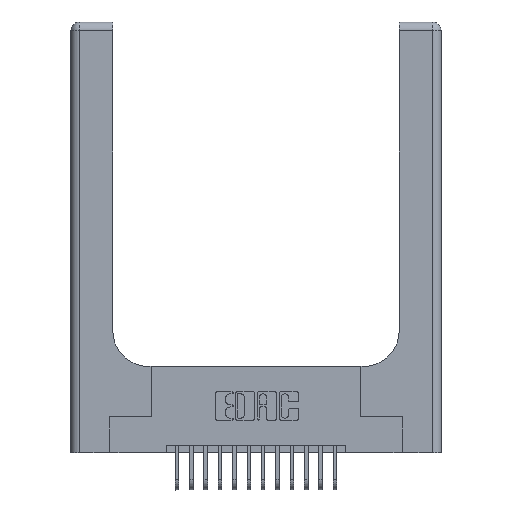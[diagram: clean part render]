
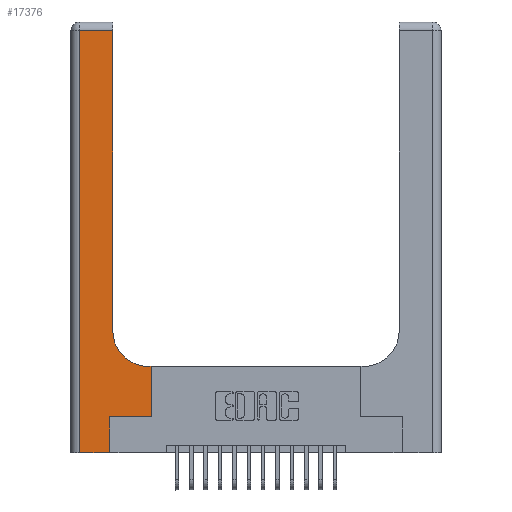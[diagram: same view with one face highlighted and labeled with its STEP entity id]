
A CAD part, top view. The second image highlights one B-rep face of the part: STEP entity #17376.
In plain terms, the highlighted planar face has unit normal (0, 0, 1).
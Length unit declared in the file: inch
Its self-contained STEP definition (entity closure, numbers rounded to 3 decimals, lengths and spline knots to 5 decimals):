
#2 = CARTESIAN_POINT ( 'NONE',  ( 0.269, 0., 0.37 ) ) ;
#33 = VERTEX_POINT ( 'NONE', #12663 ) ;
#1114 = EDGE_CURVE ( 'NONE', #33, #16928, #15766, .T. ) ;
#1162 = CARTESIAN_POINT ( 'NONE',  ( 0.5585, 0.25, 0.37 ) ) ;
#1631 = EDGE_CURVE ( 'NONE', #15964, #14121, #4961, .T. ) ;
#1657 = LINE ( 'NONE', #16995, #4989 ) ;
#2052 = DIRECTION ( 'NONE',  ( 0., -1., 0. ) ) ;
#2221 = CARTESIAN_POINT ( 'NONE',  ( 0.5585, 0.6, 0.37 ) ) ;
#2422 = VECTOR ( 'NONE', #9212, 39.37008 ) ;
#2452 = ORIENTED_EDGE ( 'NONE', *, *, #5091, .T. ) ;
#2862 = CARTESIAN_POINT ( 'NONE',  ( 0.06, 2.94, 0.37 ) ) ;
#2973 = CARTESIAN_POINT ( 'NONE',  ( 0., 2.94, 0.37 ) ) ;
#3644 = ORIENTED_EDGE ( 'NONE', *, *, #12552, .T. ) ;
#3905 = VECTOR ( 'NONE', #14409, 39.37008 ) ;
#4137 = ORIENTED_EDGE ( 'NONE', *, *, #7391, .T. ) ;
#4536 = VECTOR ( 'NONE', #15253, 39.37008 ) ;
#4923 = CARTESIAN_POINT ( 'NONE',  ( 0.06, 3., 0.37 ) ) ;
#4961 = LINE ( 'NONE', #2973, #12043 ) ;
#4989 = VECTOR ( 'NONE', #11419, 39.37008 ) ;
#5091 = EDGE_CURVE ( 'NONE', #16928, #9917, #16844, .T. ) ;
#5092 = CARTESIAN_POINT ( 'NONE',  ( 0., 3., 0.37 ) ) ;
#5603 = VECTOR ( 'NONE', #14213, 39.37008 ) ;
#5635 = DIRECTION ( 'NONE',  ( 0., 0., -1. ) ) ;
#6209 = ORIENTED_EDGE ( 'NONE', *, *, #14151, .T. ) ;
#6213 = LINE ( 'NONE', #13421, #2422 ) ;
#7259 = CARTESIAN_POINT ( 'NONE',  ( 0.5415, 0.6, 0.37 ) ) ;
#7391 = EDGE_CURVE ( 'NONE', #15913, #15964, #6213, .T. ) ;
#7506 = EDGE_LOOP ( 'NONE', ( #4137, #11533, #10899, #6209, #3644, #13629, #2452, #13275, #12934 ) ) ;
#8180 = CARTESIAN_POINT ( 'NONE',  ( 0.269, 0., 0.37 ) ) ;
#8405 = VERTEX_POINT ( 'NONE', #14320 ) ;
#9096 = LINE ( 'NONE', #4923, #16126 ) ;
#9212 = DIRECTION ( 'NONE',  ( 0., 1., 0. ) ) ;
#9365 = DIRECTION ( 'NONE',  ( -1., 0., 0. ) ) ;
#9917 = VERTEX_POINT ( 'NONE', #2221 ) ;
#10277 = CIRCLE ( 'NONE', #15326, 0.25 ) ;
#10899 = ORIENTED_EDGE ( 'NONE', *, *, #11040, .T. ) ;
#11039 = VECTOR ( 'NONE', #12853, 39.37008 ) ;
#11040 = EDGE_CURVE ( 'NONE', #14121, #8405, #9096, .T. ) ;
#11419 = DIRECTION ( 'NONE',  ( 1., 0., 0. ) ) ;
#11529 = CARTESIAN_POINT ( 'NONE',  ( 0.2915, 2.94, 0.37 ) ) ;
#11533 = ORIENTED_EDGE ( 'NONE', *, *, #1631, .T. ) ;
#12043 = VECTOR ( 'NONE', #12913, 39.37008 ) ;
#12446 = CARTESIAN_POINT ( 'NONE',  ( 0.269, 0.25, 0.37 ) ) ;
#12552 = EDGE_CURVE ( 'NONE', #17485, #33, #16068, .T. ) ;
#12606 = VERTEX_POINT ( 'NONE', #7259 ) ;
#12663 = CARTESIAN_POINT ( 'NONE',  ( 0.269, 0.25, 0.37 ) ) ;
#12853 = DIRECTION ( 'NONE',  ( 0., 1., 0. ) ) ;
#12913 = DIRECTION ( 'NONE',  ( -1., 0., 0. ) ) ;
#12934 = ORIENTED_EDGE ( 'NONE', *, *, #15863, .T. ) ;
#12990 = CARTESIAN_POINT ( 'NONE',  ( 0.2915, 0.6, 0.37 ) ) ;
#13275 = ORIENTED_EDGE ( 'NONE', *, *, #13519, .T. ) ;
#13421 = CARTESIAN_POINT ( 'NONE',  ( 0.2915, 3., 0.37 ) ) ;
#13519 = EDGE_CURVE ( 'NONE', #9917, #12606, #15182, .T. ) ;
#13629 = ORIENTED_EDGE ( 'NONE', *, *, #1114, .T. ) ;
#14121 = VERTEX_POINT ( 'NONE', #2862 ) ;
#14125 = CARTESIAN_POINT ( 'NONE',  ( 0.5415, 0.85, 0.37 ) ) ;
#14151 = EDGE_CURVE ( 'NONE', #8405, #17485, #1657, .T. ) ;
#14213 = DIRECTION ( 'NONE',  ( 0., 1., 0. ) ) ;
#14320 = CARTESIAN_POINT ( 'NONE',  ( 0.06, 0., 0.37 ) ) ;
#14409 = DIRECTION ( 'NONE',  ( -1., 0., 0. ) ) ;
#14984 = PLANE ( 'NONE',  #18261 ) ;
#15182 = LINE ( 'NONE', #12990, #3905 ) ;
#15253 = DIRECTION ( 'NONE',  ( 1., 0., 0. ) ) ;
#15326 = AXIS2_PLACEMENT_3D ( 'NONE', #14125, #5635, #15507 ) ;
#15507 = DIRECTION ( 'NONE',  ( 1., 0., 0. ) ) ;
#15766 = LINE ( 'NONE', #12446, #4536 ) ;
#15863 = EDGE_CURVE ( 'NONE', #12606, #15913, #10277, .T. ) ;
#15913 = VERTEX_POINT ( 'NONE', #16982 ) ;
#15964 = VERTEX_POINT ( 'NONE', #11529 ) ;
#16068 = LINE ( 'NONE', #2, #11039 ) ;
#16126 = VECTOR ( 'NONE', #2052, 39.37008 ) ;
#16844 = LINE ( 'NONE', #18331, #5603 ) ;
#16928 = VERTEX_POINT ( 'NONE', #1162 ) ;
#16982 = CARTESIAN_POINT ( 'NONE',  ( 0.2915, 0.85, 0.37 ) ) ;
#16995 = CARTESIAN_POINT ( 'NONE',  ( 0., 0., 0.37 ) ) ;
#17272 = FACE_OUTER_BOUND ( 'NONE', #7506, .T. ) ;
#17376 = ADVANCED_FACE ( 'NONE', ( #17272 ), #14984, .F. ) ;
#17485 = VERTEX_POINT ( 'NONE', #8180 ) ;
#17764 = DIRECTION ( 'NONE',  ( 0., 0., -1. ) ) ;
#18261 = AXIS2_PLACEMENT_3D ( 'NONE', #5092, #17764, #9365 ) ;
#18331 = CARTESIAN_POINT ( 'NONE',  ( 0.5585, 0.25, 0.37 ) ) ;
